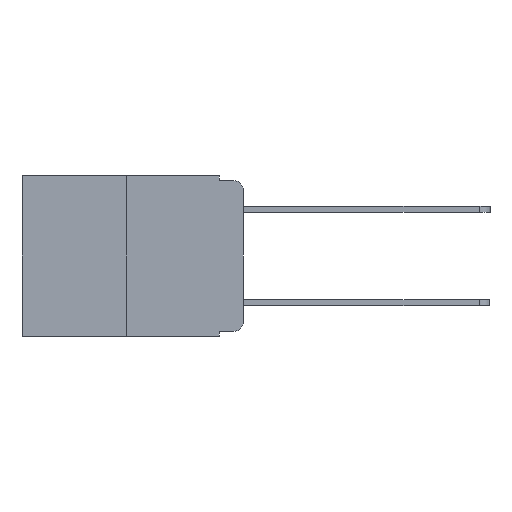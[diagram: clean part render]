
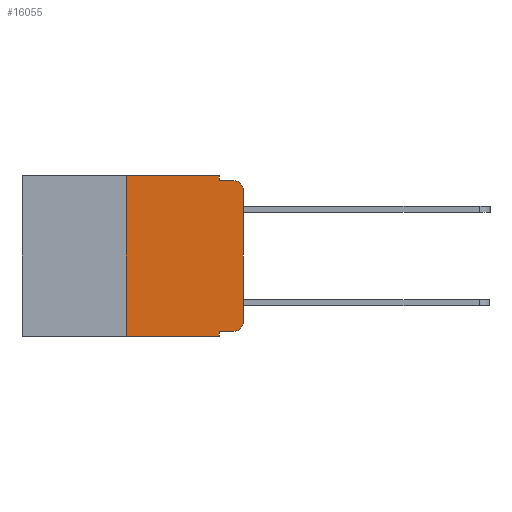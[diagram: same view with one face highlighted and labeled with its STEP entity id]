
A CAD part, left-side view. The second image highlights one B-rep face of the part: STEP entity #16055.
In plain terms, the highlighted planar face has unit normal (-1, 0, 0).
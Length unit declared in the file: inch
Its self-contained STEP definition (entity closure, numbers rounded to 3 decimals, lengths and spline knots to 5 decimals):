
#162 = VERTEX_POINT ( 'NONE', #6943 ) ;
#653 = EDGE_CURVE ( 'NONE', #10170, #14324, #1640, .T. ) ;
#1213 = VERTEX_POINT ( 'NONE', #16438 ) ;
#1455 = CARTESIAN_POINT ( 'NONE',  ( 0., 0.051, 0. ) ) ;
#1640 = LINE ( 'NONE', #10878, #12708 ) ;
#1742 = PLANE ( 'NONE',  #5960 ) ;
#2100 = CARTESIAN_POINT ( 'NONE',  ( 0., 0.02, -0.03 ) ) ;
#2374 = VECTOR ( 'NONE', #17863, 39.37008 ) ;
#2871 = DIRECTION ( 'NONE',  ( -1., 0., 0. ) ) ;
#2876 = VERTEX_POINT ( 'NONE', #3424 ) ;
#2926 = CARTESIAN_POINT ( 'NONE',  ( 0., 0.02, -0.01 ) ) ;
#2961 = ORIENTED_EDGE ( 'NONE', *, *, #16601, .F. ) ;
#3197 = ORIENTED_EDGE ( 'NONE', *, *, #9811, .T. ) ;
#3211 = CARTESIAN_POINT ( 'NONE',  ( 0., 0., 0. ) ) ;
#3217 = ORIENTED_EDGE ( 'NONE', *, *, #14389, .T. ) ;
#3244 = VECTOR ( 'NONE', #13009, 39.37008 ) ;
#3424 = CARTESIAN_POINT ( 'NONE',  ( 0., 0., -0.313 ) ) ;
#3645 = CARTESIAN_POINT ( 'NONE',  ( 0., 0.02, -0.333 ) ) ;
#3669 = DIRECTION ( 'NONE',  ( 0., 0., -1. ) ) ;
#4607 = EDGE_CURVE ( 'NONE', #6883, #14420, #17395, .T. ) ;
#4848 = DIRECTION ( 'NONE',  ( 1., 0., 0. ) ) ;
#4895 = CIRCLE ( 'NONE', #15103, 0.02 ) ;
#5013 = VECTOR ( 'NONE', #11636, 39.37008 ) ;
#5233 = VECTOR ( 'NONE', #17065, 39.37008 ) ;
#5468 = AXIS2_PLACEMENT_3D ( 'NONE', #2100, #12190, #3669 ) ;
#5514 = ORIENTED_EDGE ( 'NONE', *, *, #17291, .T. ) ;
#5734 = DIRECTION ( 'NONE',  ( 0., 0., 1. ) ) ;
#5818 = ORIENTED_EDGE ( 'NONE', *, *, #17120, .T. ) ;
#5960 = AXIS2_PLACEMENT_3D ( 'NONE', #13254, #4848, #14609 ) ;
#6129 = LINE ( 'NONE', #3211, #13117 ) ;
#6234 = DIRECTION ( 'NONE',  ( 0., -1., 0. ) ) ;
#6612 = ORIENTED_EDGE ( 'NONE', *, *, #7719, .T. ) ;
#6883 = VERTEX_POINT ( 'NONE', #14028 ) ;
#6923 = VERTEX_POINT ( 'NONE', #15441 ) ;
#6943 = CARTESIAN_POINT ( 'NONE',  ( 0., 0.25, 0. ) ) ;
#7491 = EDGE_CURVE ( 'NONE', #9085, #162, #14546, .T. ) ;
#7719 = EDGE_CURVE ( 'NONE', #2876, #6923, #6129, .T. ) ;
#7744 = EDGE_LOOP ( 'NONE', ( #6612, #5514, #8419, #2961, #8649, #9776, #3197, #11521, #3217, #5818 ) ) ;
#8419 = ORIENTED_EDGE ( 'NONE', *, *, #653, .F. ) ;
#8649 = ORIENTED_EDGE ( 'NONE', *, *, #13167, .F. ) ;
#8927 = CARTESIAN_POINT ( 'NONE',  ( 0., 0.051, -0.343 ) ) ;
#9085 = VERTEX_POINT ( 'NONE', #12983 ) ;
#9457 = LINE ( 'NONE', #10277, #5233 ) ;
#9776 = ORIENTED_EDGE ( 'NONE', *, *, #7491, .F. ) ;
#9811 = EDGE_CURVE ( 'NONE', #9085, #14420, #18344, .T. ) ;
#10170 = VERTEX_POINT ( 'NONE', #18096 ) ;
#10277 = CARTESIAN_POINT ( 'NONE',  ( 0., 0.051, -0.333 ) ) ;
#10434 = CARTESIAN_POINT ( 'NONE',  ( 0., 0.473, -0.343 ) ) ;
#10878 = CARTESIAN_POINT ( 'NONE',  ( 0., 0.051, -0.01 ) ) ;
#11487 = CARTESIAN_POINT ( 'NONE',  ( 0., 0.02, -0.313 ) ) ;
#11521 = ORIENTED_EDGE ( 'NONE', *, *, #4607, .F. ) ;
#11636 = DIRECTION ( 'NONE',  ( 0., -1., 0. ) ) ;
#12190 = DIRECTION ( 'NONE',  ( -1., 0., 0. ) ) ;
#12708 = VECTOR ( 'NONE', #17991, 39.37008 ) ;
#12878 = DIRECTION ( 'NONE',  ( 0., 0., -1. ) ) ;
#12983 = CARTESIAN_POINT ( 'NONE',  ( 0., 0.25, -0.343 ) ) ;
#13009 = DIRECTION ( 'NONE',  ( 0., 0., -1. ) ) ;
#13117 = VECTOR ( 'NONE', #14586, 39.37008 ) ;
#13167 = EDGE_CURVE ( 'NONE', #162, #1213, #15691, .T. ) ;
#13254 = CARTESIAN_POINT ( 'NONE',  ( 0., 0.473, 0. ) ) ;
#14028 = CARTESIAN_POINT ( 'NONE',  ( 0., 0.051, -0.333 ) ) ;
#14110 = LINE ( 'NONE', #1455, #3244 ) ;
#14125 = VECTOR ( 'NONE', #5734, 39.37008 ) ;
#14324 = VERTEX_POINT ( 'NONE', #2926 ) ;
#14389 = EDGE_CURVE ( 'NONE', #6883, #17938, #9457, .T. ) ;
#14420 = VERTEX_POINT ( 'NONE', #8927 ) ;
#14546 = LINE ( 'NONE', #15414, #14125 ) ;
#14586 = DIRECTION ( 'NONE',  ( 0., 0., 1. ) ) ;
#14609 = DIRECTION ( 'NONE',  ( 0., 0., -1. ) ) ;
#14702 = VECTOR ( 'NONE', #6234, 39.37008 ) ;
#15045 = CARTESIAN_POINT ( 'NONE',  ( 0., 0.051, 0. ) ) ;
#15103 = AXIS2_PLACEMENT_3D ( 'NONE', #11487, #2871, #12878 ) ;
#15414 = CARTESIAN_POINT ( 'NONE',  ( 0., 0.25, 0. ) ) ;
#15441 = CARTESIAN_POINT ( 'NONE',  ( 0., 0., -0.03 ) ) ;
#15691 = LINE ( 'NONE', #18411, #5013 ) ;
#16055 = ADVANCED_FACE ( 'NONE', ( #16250 ), #1742, .F. ) ;
#16192 = CIRCLE ( 'NONE', #5468, 0.02 ) ;
#16250 = FACE_OUTER_BOUND ( 'NONE', #7744, .T. ) ;
#16438 = CARTESIAN_POINT ( 'NONE',  ( 0., 0.051, 0. ) ) ;
#16601 = EDGE_CURVE ( 'NONE', #1213, #10170, #14110, .T. ) ;
#17065 = DIRECTION ( 'NONE',  ( 0., -1., 0. ) ) ;
#17120 = EDGE_CURVE ( 'NONE', #17938, #2876, #4895, .T. ) ;
#17291 = EDGE_CURVE ( 'NONE', #6923, #14324, #16192, .T. ) ;
#17395 = LINE ( 'NONE', #15045, #2374 ) ;
#17863 = DIRECTION ( 'NONE',  ( 0., 0., -1. ) ) ;
#17938 = VERTEX_POINT ( 'NONE', #3645 ) ;
#17991 = DIRECTION ( 'NONE',  ( 0., -1., 0. ) ) ;
#18096 = CARTESIAN_POINT ( 'NONE',  ( 0., 0.051, -0.01 ) ) ;
#18344 = LINE ( 'NONE', #10434, #14702 ) ;
#18411 = CARTESIAN_POINT ( 'NONE',  ( 0., 0.473, 0. ) ) ;
